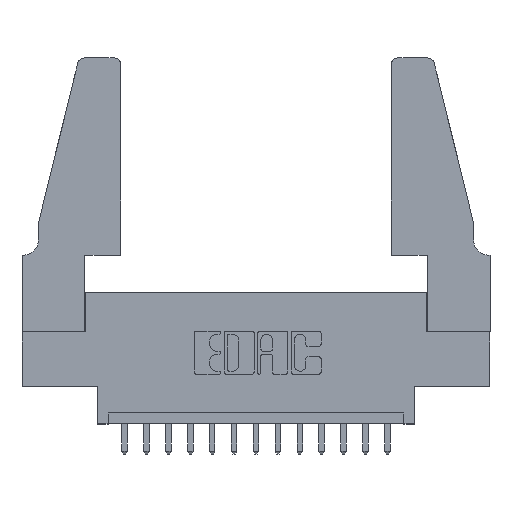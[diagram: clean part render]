
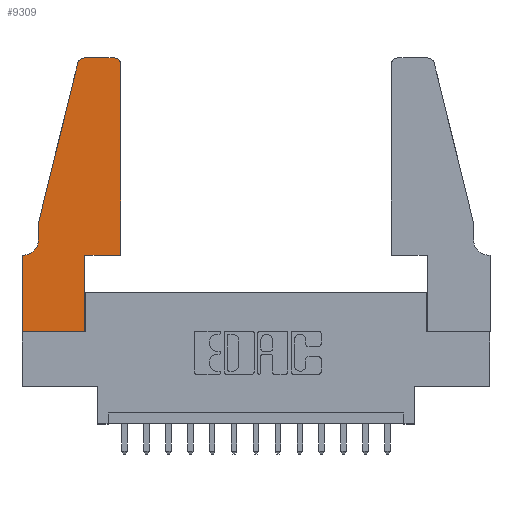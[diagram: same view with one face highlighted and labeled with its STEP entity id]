
A CAD part, top view. The second image highlights one B-rep face of the part: STEP entity #9309.
In plain terms, the highlighted planar face has unit normal (0, 0, 1).
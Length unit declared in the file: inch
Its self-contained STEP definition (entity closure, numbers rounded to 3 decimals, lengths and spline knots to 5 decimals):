
#109 = EDGE_CURVE ( 'NONE', #11398, #13244, #9382, .T. ) ;
#254 = DIRECTION ( 'NONE',  ( 1., 0., 0. ) ) ;
#290 = DIRECTION ( 'NONE',  ( -0.239, -0.971, 0. ) ) ;
#323 = CARTESIAN_POINT ( 'NONE',  ( 0., 0.35, 0.37 ) ) ;
#510 = CARTESIAN_POINT ( 'NONE',  ( 0.4205, 1.22, 0.37 ) ) ;
#886 = EDGE_LOOP ( 'NONE', ( #3692, #10619, #12015, #9606, #8686, #10866, #6736, #1703, #4115, #7051, #6051, #1123 ) ) ;
#971 = LINE ( 'NONE', #15023, #13722 ) ;
#1123 = ORIENTED_EDGE ( 'NONE', *, *, #1882, .T. ) ;
#1276 = VERTEX_POINT ( 'NONE', #5019 ) ;
#1458 = EDGE_CURVE ( 'NONE', #9159, #14909, #9932, .T. ) ;
#1469 = CARTESIAN_POINT ( 'NONE',  ( 0.4205, 1.25, 0.37 ) ) ;
#1703 = ORIENTED_EDGE ( 'NONE', *, *, #12537, .T. ) ;
#1771 = DIRECTION ( 'NONE',  ( 0., -1., 0. ) ) ;
#1882 = EDGE_CURVE ( 'NONE', #6042, #6154, #11890, .T. ) ;
#1967 = DIRECTION ( 'NONE',  ( 0., 0., 1. ) ) ;
#2133 = FACE_OUTER_BOUND ( 'NONE', #886, .T. ) ;
#2266 = DIRECTION ( 'NONE',  ( 1., 0., 0. ) ) ;
#2678 = EDGE_CURVE ( 'NONE', #5229, #9159, #10978, .T. ) ;
#2696 = LINE ( 'NONE', #15802, #9131 ) ;
#2759 = CARTESIAN_POINT ( 'NONE',  ( 0., 0.35, 0.37 ) ) ;
#3137 = DIRECTION ( 'NONE',  ( -1., 0., 0. ) ) ;
#3149 = CARTESIAN_POINT ( 'NONE',  ( 0.25487, 1.22718, 0.37 ) ) ;
#3161 = EDGE_CURVE ( 'NONE', #14909, #5427, #4968, .T. ) ;
#3247 = EDGE_CURVE ( 'NONE', #5427, #13568, #7700, .T. ) ;
#3692 = ORIENTED_EDGE ( 'NONE', *, *, #6790, .T. ) ;
#4115 = ORIENTED_EDGE ( 'NONE', *, *, #10732, .T. ) ;
#4321 = DIRECTION ( 'NONE',  ( 0., 1., 0. ) ) ;
#4443 = CARTESIAN_POINT ( 'NONE',  ( 0.0055, 0.42, 0.37 ) ) ;
#4599 = VERTEX_POINT ( 'NONE', #10839 ) ;
#4820 = CARTESIAN_POINT ( 'NONE',  ( 0.284, 1.25, 0.37 ) ) ;
#4824 = CARTESIAN_POINT ( 'NONE',  ( 0.0055, 0.35, 0.37 ) ) ;
#4968 = LINE ( 'NONE', #11211, #14467 ) ;
#5019 = CARTESIAN_POINT ( 'NONE',  ( 0.2865, 0.35, 0.37 ) ) ;
#5228 = VECTOR ( 'NONE', #4321, 39.37008 ) ;
#5229 = VERTEX_POINT ( 'NONE', #15516 ) ;
#5258 = CARTESIAN_POINT ( 'NONE',  ( 0., 0., 0.37 ) ) ;
#5317 = CARTESIAN_POINT ( 'NONE',  ( 0.284, 1.22, 0.37 ) ) ;
#5427 = VERTEX_POINT ( 'NONE', #323 ) ;
#6042 = VERTEX_POINT ( 'NONE', #12292 ) ;
#6051 = ORIENTED_EDGE ( 'NONE', *, *, #15475, .T. ) ;
#6154 = VERTEX_POINT ( 'NONE', #1469 ) ;
#6285 = DIRECTION ( 'NONE',  ( 0., 1., 0. ) ) ;
#6736 = ORIENTED_EDGE ( 'NONE', *, *, #3247, .T. ) ;
#6790 = EDGE_CURVE ( 'NONE', #6154, #11398, #12798, .T. ) ;
#6983 = CARTESIAN_POINT ( 'NONE',  ( 0.2865, 0., 0.37 ) ) ;
#7051 = ORIENTED_EDGE ( 'NONE', *, *, #15782, .T. ) ;
#7418 = DIRECTION ( 'NONE',  ( 0., 0., 1. ) ) ;
#7465 = EDGE_CURVE ( 'NONE', #13244, #5229, #971, .T. ) ;
#7600 = CARTESIAN_POINT ( 'NONE',  ( 0., 0., 0.37 ) ) ;
#7700 = LINE ( 'NONE', #7600, #10616 ) ;
#7755 = LINE ( 'NONE', #11771, #5228 ) ;
#8033 = CARTESIAN_POINT ( 'NONE',  ( 0.2865, 0.35, 0.37 ) ) ;
#8131 = VECTOR ( 'NONE', #6285, 39.37008 ) ;
#8608 = AXIS2_PLACEMENT_3D ( 'NONE', #4443, #11788, #13080 ) ;
#8686 = ORIENTED_EDGE ( 'NONE', *, *, #1458, .T. ) ;
#9083 = DIRECTION ( 'NONE',  ( 0., 0., 1. ) ) ;
#9131 = VECTOR ( 'NONE', #13107, 39.37008 ) ;
#9159 = VERTEX_POINT ( 'NONE', #11715 ) ;
#9309 = ADVANCED_FACE ( 'NONE', ( #2133 ), #15314, .T. ) ;
#9382 = CIRCLE ( 'NONE', #14348, 0.03 ) ;
#9547 = VECTOR ( 'NONE', #3137, 39.37008 ) ;
#9606 = ORIENTED_EDGE ( 'NONE', *, *, #2678, .T. ) ;
#9932 = CIRCLE ( 'NONE', #8608, 0.07 ) ;
#10293 = VERTEX_POINT ( 'NONE', #6983 ) ;
#10616 = VECTOR ( 'NONE', #12722, 39.37008 ) ;
#10619 = ORIENTED_EDGE ( 'NONE', *, *, #109, .T. ) ;
#10638 = DIRECTION ( 'NONE',  ( 1., 0., 0. ) ) ;
#10732 = EDGE_CURVE ( 'NONE', #10293, #1276, #11387, .T. ) ;
#10839 = CARTESIAN_POINT ( 'NONE',  ( 0.4505, 0.35, 0.37 ) ) ;
#10866 = ORIENTED_EDGE ( 'NONE', *, *, #3161, .T. ) ;
#10978 = LINE ( 'NONE', #11391, #13293 ) ;
#11211 = CARTESIAN_POINT ( 'NONE',  ( 0.0755, 0.35, 0.37 ) ) ;
#11387 = LINE ( 'NONE', #8033, #8131 ) ;
#11391 = CARTESIAN_POINT ( 'NONE',  ( 0.0755, 0.5, 0.37 ) ) ;
#11398 = VERTEX_POINT ( 'NONE', #4820 ) ;
#11418 = AXIS2_PLACEMENT_3D ( 'NONE', #2759, #7418, #2266 ) ;
#11715 = CARTESIAN_POINT ( 'NONE',  ( 0.0755, 0.42, 0.37 ) ) ;
#11771 = CARTESIAN_POINT ( 'NONE',  ( 0.4505, 0.35, 0.37 ) ) ;
#11788 = DIRECTION ( 'NONE',  ( 0., 0., -1. ) ) ;
#11890 = CIRCLE ( 'NONE', #11980, 0.03 ) ;
#11980 = AXIS2_PLACEMENT_3D ( 'NONE', #510, #1967, #10638 ) ;
#12015 = ORIENTED_EDGE ( 'NONE', *, *, #7465, .T. ) ;
#12292 = CARTESIAN_POINT ( 'NONE',  ( 0.4505, 1.22, 0.37 ) ) ;
#12537 = EDGE_CURVE ( 'NONE', #13568, #10293, #15362, .T. ) ;
#12722 = DIRECTION ( 'NONE',  ( 0., -1., 0. ) ) ;
#12798 = LINE ( 'NONE', #13963, #9547 ) ;
#13080 = DIRECTION ( 'NONE',  ( -1., 0., 0. ) ) ;
#13107 = DIRECTION ( 'NONE',  ( 1., 0., 0. ) ) ;
#13244 = VERTEX_POINT ( 'NONE', #3149 ) ;
#13293 = VECTOR ( 'NONE', #1771, 39.37008 ) ;
#13568 = VERTEX_POINT ( 'NONE', #5258 ) ;
#13722 = VECTOR ( 'NONE', #290, 39.37008 ) ;
#13963 = CARTESIAN_POINT ( 'NONE',  ( 0.2605, 1.25, 0.37 ) ) ;
#14145 = DIRECTION ( 'NONE',  ( 1., 0., 0. ) ) ;
#14348 = AXIS2_PLACEMENT_3D ( 'NONE', #5317, #9083, #254 ) ;
#14467 = VECTOR ( 'NONE', #14872, 39.37008 ) ;
#14872 = DIRECTION ( 'NONE',  ( -1., 0., 0. ) ) ;
#14909 = VERTEX_POINT ( 'NONE', #4824 ) ;
#15023 = CARTESIAN_POINT ( 'NONE',  ( 0.0755, 0.5, 0.37 ) ) ;
#15314 = PLANE ( 'NONE',  #11418 ) ;
#15362 = LINE ( 'NONE', #15382, #15761 ) ;
#15382 = CARTESIAN_POINT ( 'NONE',  ( 0., 0., 0.37 ) ) ;
#15475 = EDGE_CURVE ( 'NONE', #4599, #6042, #7755, .T. ) ;
#15516 = CARTESIAN_POINT ( 'NONE',  ( 0.0755, 0.5, 0.37 ) ) ;
#15761 = VECTOR ( 'NONE', #14145, 39.37008 ) ;
#15782 = EDGE_CURVE ( 'NONE', #1276, #4599, #2696, .T. ) ;
#15802 = CARTESIAN_POINT ( 'NONE',  ( 0.4505, 0.35, 0.37 ) ) ;
